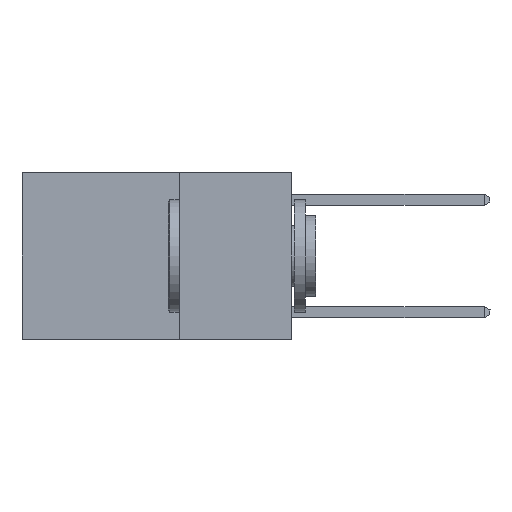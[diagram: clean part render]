
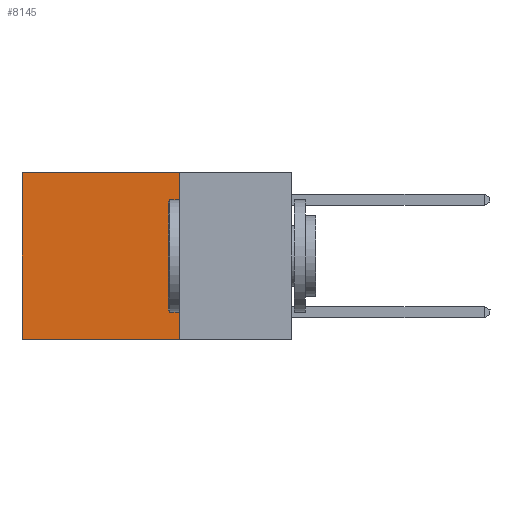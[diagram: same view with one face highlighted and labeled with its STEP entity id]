
A CAD part, left-side view. The second image highlights one B-rep face of the part: STEP entity #8145.
In plain terms, the highlighted planar face has unit normal (-1, 0, 0).
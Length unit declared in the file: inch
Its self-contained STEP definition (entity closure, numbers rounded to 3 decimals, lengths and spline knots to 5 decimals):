
#1755 = LINE ( 'NONE', #4727, #31402 ) ;
#1921 = DIRECTION ( 'NONE',  ( 0., 0., -1. ) ) ;
#3191 = VECTOR ( 'NONE', #22182, 39.37008 ) ;
#4483 = EDGE_CURVE ( 'NONE', #29583, #9368, #20878, .T. ) ;
#4727 = CARTESIAN_POINT ( 'NONE',  ( 0.2625, 0.6, 0. ) ) ;
#5298 = AXIS2_PLACEMENT_3D ( 'NONE', #19857, #20188, #32287 ) ;
#5936 = VERTEX_POINT ( 'NONE', #27058 ) ;
#6117 = EDGE_LOOP ( 'NONE', ( #12124, #28966, #19091, #31356 ) ) ;
#7471 = CARTESIAN_POINT ( 'NONE',  ( 0.2625, 0.25, 0. ) ) ;
#8145 = ADVANCED_FACE ( 'NONE', ( #10114 ), #17235, .F. ) ;
#9368 = VERTEX_POINT ( 'NONE', #16116 ) ;
#10114 = FACE_OUTER_BOUND ( 'NONE', #6117, .T. ) ;
#12124 = ORIENTED_EDGE ( 'NONE', *, *, #14252, .T. ) ;
#14252 = EDGE_CURVE ( 'NONE', #25311, #9368, #1755, .T. ) ;
#16116 = CARTESIAN_POINT ( 'NONE',  ( 0.2625, 0.6, -0.37 ) ) ;
#16230 = DIRECTION ( 'NONE',  ( 0., 1., 0. ) ) ;
#16529 = VECTOR ( 'NONE', #27981, 39.37008 ) ;
#17235 = PLANE ( 'NONE',  #5298 ) ;
#19091 = ORIENTED_EDGE ( 'NONE', *, *, #24640, .F. ) ;
#19677 = LINE ( 'NONE', #24981, #3191 ) ;
#19857 = CARTESIAN_POINT ( 'NONE',  ( 0.2625, 0.25, 0. ) ) ;
#20188 = DIRECTION ( 'NONE',  ( 1., 0., 0. ) ) ;
#20878 = LINE ( 'NONE', #31304, #26557 ) ;
#22182 = DIRECTION ( 'NONE',  ( 0., 0., -1. ) ) ;
#24640 = EDGE_CURVE ( 'NONE', #5936, #29583, #19677, .T. ) ;
#24981 = CARTESIAN_POINT ( 'NONE',  ( 0.2625, 0.25, 0. ) ) ;
#25311 = VERTEX_POINT ( 'NONE', #30558 ) ;
#25512 = CARTESIAN_POINT ( 'NONE',  ( 0.2625, 0.25, -0.37 ) ) ;
#26557 = VECTOR ( 'NONE', #16230, 39.37008 ) ;
#27058 = CARTESIAN_POINT ( 'NONE',  ( 0.2625, 0.25, 0. ) ) ;
#27950 = EDGE_CURVE ( 'NONE', #5936, #25311, #32447, .T. ) ;
#27981 = DIRECTION ( 'NONE',  ( 0., 1., 0. ) ) ;
#28966 = ORIENTED_EDGE ( 'NONE', *, *, #4483, .F. ) ;
#29583 = VERTEX_POINT ( 'NONE', #25512 ) ;
#30558 = CARTESIAN_POINT ( 'NONE',  ( 0.2625, 0.6, 0. ) ) ;
#31304 = CARTESIAN_POINT ( 'NONE',  ( 0.2625, 0.25, -0.37 ) ) ;
#31356 = ORIENTED_EDGE ( 'NONE', *, *, #27950, .T. ) ;
#31402 = VECTOR ( 'NONE', #1921, 39.37008 ) ;
#32287 = DIRECTION ( 'NONE',  ( 0., 0., -1. ) ) ;
#32447 = LINE ( 'NONE', #7471, #16529 ) ;
